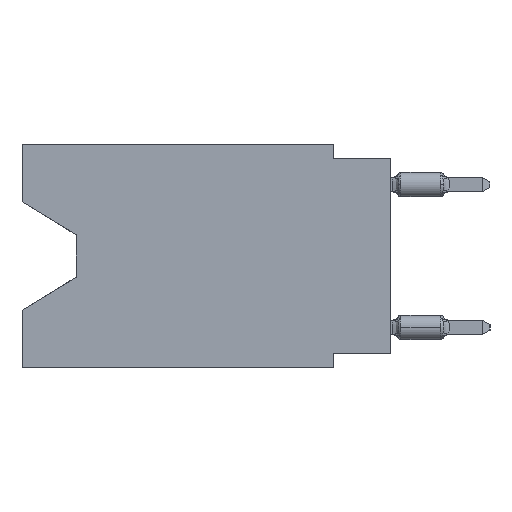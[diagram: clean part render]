
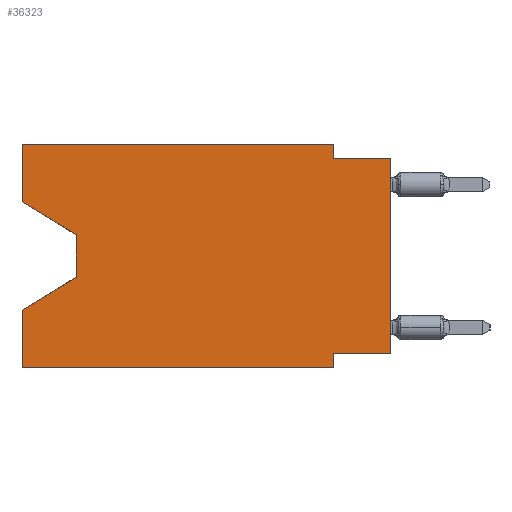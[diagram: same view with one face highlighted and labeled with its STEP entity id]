
A CAD part, left-side view. The second image highlights one B-rep face of the part: STEP entity #36323.
In plain terms, the highlighted planar face has unit normal (-1, 0, 0).
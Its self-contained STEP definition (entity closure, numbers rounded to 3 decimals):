
#800 = CARTESIAN_POINT ( 'NONE',  ( 0., 16.383, 0. ) ) ;
#2239 = LINE ( 'NONE', #11831, #48342 ) ;
#5700 = CARTESIAN_POINT ( 'NONE',  ( 0., 0., -0.635 ) ) ;
#6892 = CARTESIAN_POINT ( 'NONE',  ( 0., 16.383, 0. ) ) ;
#7285 = EDGE_CURVE ( 'NONE', #55213, #67198, #36756, .T. ) ;
#11448 = DIRECTION ( 'NONE',  ( 0., 0., -1. ) ) ;
#11802 = CARTESIAN_POINT ( 'NONE',  ( 0., 13.97, -5.893 ) ) ;
#11831 = CARTESIAN_POINT ( 'NONE',  ( 0., 0., 0. ) ) ;
#11960 = DIRECTION ( 'NONE',  ( 0., -1., 0. ) ) ;
#12684 = EDGE_CURVE ( 'NONE', #23240, #52207, #2239, .T. ) ;
#12736 = DIRECTION ( 'NONE',  ( 0., 1., 0. ) ) ;
#13069 = CARTESIAN_POINT ( 'NONE',  ( 0., 0., -9.271 ) ) ;
#14661 = VECTOR ( 'NONE', #11448, 1000. ) ;
#14761 = VECTOR ( 'NONE', #53350, 1000. ) ;
#14791 = VECTOR ( 'NONE', #12736, 1000. ) ;
#15826 = EDGE_CURVE ( 'NONE', #63662, #47888, #22528, .T. ) ;
#17516 = DIRECTION ( 'NONE',  ( 1., 0., 0. ) ) ;
#18167 = CARTESIAN_POINT ( 'NONE',  ( 0., 0., -0.635 ) ) ;
#18464 = VECTOR ( 'NONE', #56371, 1000. ) ;
#18908 = VECTOR ( 'NONE', #11960, 1000. ) ;
#19835 = VERTEX_POINT ( 'NONE', #65864 ) ;
#21396 = ORIENTED_EDGE ( 'NONE', *, *, #31389, .F. ) ;
#21735 = CARTESIAN_POINT ( 'NONE',  ( 0., 2.54, -9.906 ) ) ;
#22528 = LINE ( 'NONE', #32467, #14761 ) ;
#22677 = LINE ( 'NONE', #800, #52258 ) ;
#23240 = VERTEX_POINT ( 'NONE', #43966 ) ;
#23851 = CARTESIAN_POINT ( 'NONE',  ( 0., 13.97, -5.893 ) ) ;
#24217 = CARTESIAN_POINT ( 'NONE',  ( 0., 13.97, -4.013 ) ) ;
#25348 = EDGE_LOOP ( 'NONE', ( #44290, #29665, #33543, #37203, #29110, #52656, #36316, #64169, #21396, #58352, #28528, #28269 ) ) ;
#25919 = VERTEX_POINT ( 'NONE', #48844 ) ;
#27871 = LINE ( 'NONE', #37817, #14661 ) ;
#28008 = EDGE_CURVE ( 'NONE', #23240, #52487, #64433, .T. ) ;
#28269 = ORIENTED_EDGE ( 'NONE', *, *, #47150, .F. ) ;
#28528 = ORIENTED_EDGE ( 'NONE', *, *, #7285, .F. ) ;
#29110 = ORIENTED_EDGE ( 'NONE', *, *, #40261, .T. ) ;
#29665 = ORIENTED_EDGE ( 'NONE', *, *, #15826, .T. ) ;
#29707 = VECTOR ( 'NONE', #60527, 1000. ) ;
#31389 = EDGE_CURVE ( 'NONE', #46393, #52207, #39395, .T. ) ;
#31607 = CARTESIAN_POINT ( 'NONE',  ( 0., 16.383, 0. ) ) ;
#32467 = CARTESIAN_POINT ( 'NONE',  ( 0., 13.97, -4.013 ) ) ;
#32497 = VECTOR ( 'NONE', #43721, 1000. ) ;
#32940 = DIRECTION ( 'NONE',  ( 0., 0., 1. ) ) ;
#33543 = ORIENTED_EDGE ( 'NONE', *, *, #49444, .T. ) ;
#33613 = CARTESIAN_POINT ( 'NONE',  ( 0., 16.383, 0. ) ) ;
#33889 = EDGE_CURVE ( 'NONE', #19835, #63662, #44783, .T. ) ;
#34357 = CARTESIAN_POINT ( 'NONE',  ( 0., 16.383, -7.36 ) ) ;
#35207 = LINE ( 'NONE', #56763, #59615 ) ;
#35753 = VERTEX_POINT ( 'NONE', #21735 ) ;
#36316 = ORIENTED_EDGE ( 'NONE', *, *, #28008, .F. ) ;
#36323 = ADVANCED_FACE ( 'NONE', ( #38090 ), #58961, .F. ) ;
#36756 = LINE ( 'NONE', #31607, #66959 ) ;
#37203 = ORIENTED_EDGE ( 'NONE', *, *, #61105, .F. ) ;
#37817 = CARTESIAN_POINT ( 'NONE',  ( 0., 2.54, 0. ) ) ;
#37995 = CARTESIAN_POINT ( 'NONE',  ( 0., 16.383, -9.906 ) ) ;
#38090 = FACE_OUTER_BOUND ( 'NONE', #25348, .T. ) ;
#39395 = LINE ( 'NONE', #18167, #67564 ) ;
#40261 = EDGE_CURVE ( 'NONE', #25919, #35753, #58865, .T. ) ;
#41726 = EDGE_CURVE ( 'NONE', #67198, #46393, #27871, .T. ) ;
#43721 = DIRECTION ( 'NONE',  ( 0., 0.855, -0.519 ) ) ;
#43856 = DIRECTION ( 'NONE',  ( 0., -1., 0. ) ) ;
#43966 = CARTESIAN_POINT ( 'NONE',  ( 0., 0., -9.271 ) ) ;
#44290 = ORIENTED_EDGE ( 'NONE', *, *, #33889, .T. ) ;
#44783 = LINE ( 'NONE', #65651, #29707 ) ;
#46393 = VERTEX_POINT ( 'NONE', #66174 ) ;
#47150 = EDGE_CURVE ( 'NONE', #19835, #55213, #35207, .T. ) ;
#47888 = VERTEX_POINT ( 'NONE', #11802 ) ;
#48342 = VECTOR ( 'NONE', #64863, 1000. ) ;
#48371 = DIRECTION ( 'NONE',  ( 0., -1., 0. ) ) ;
#48844 = CARTESIAN_POINT ( 'NONE',  ( 0., 16.383, -9.906 ) ) ;
#49444 = EDGE_CURVE ( 'NONE', #47888, #59619, #59459, .T. ) ;
#52207 = VERTEX_POINT ( 'NONE', #5700 ) ;
#52258 = VECTOR ( 'NONE', #32940, 1000. ) ;
#52487 = VERTEX_POINT ( 'NONE', #61425 ) ;
#52656 = ORIENTED_EDGE ( 'NONE', *, *, #62608, .F. ) ;
#53350 = DIRECTION ( 'NONE',  ( 0., 0., -1. ) ) ;
#54489 = DIRECTION ( 'NONE',  ( 0., 0., -1. ) ) ;
#55213 = VERTEX_POINT ( 'NONE', #6892 ) ;
#56371 = DIRECTION ( 'NONE',  ( 0., 0., -1. ) ) ;
#56763 = CARTESIAN_POINT ( 'NONE',  ( 0., 16.383, 0. ) ) ;
#58352 = ORIENTED_EDGE ( 'NONE', *, *, #41726, .F. ) ;
#58865 = LINE ( 'NONE', #37995, #18908 ) ;
#58961 = PLANE ( 'NONE',  #64783 ) ;
#59459 = LINE ( 'NONE', #23851, #32497 ) ;
#59615 = VECTOR ( 'NONE', #61555, 1000. ) ;
#59619 = VERTEX_POINT ( 'NONE', #34357 ) ;
#60527 = DIRECTION ( 'NONE',  ( 0., -0.855, -0.519 ) ) ;
#61105 = EDGE_CURVE ( 'NONE', #25919, #59619, #22677, .T. ) ;
#61195 = CARTESIAN_POINT ( 'NONE',  ( 0., 2.54, 0. ) ) ;
#61425 = CARTESIAN_POINT ( 'NONE',  ( 0., 2.54, -9.271 ) ) ;
#61555 = DIRECTION ( 'NONE',  ( 0., 0., 1. ) ) ;
#61842 = CARTESIAN_POINT ( 'NONE',  ( 0., 2.54, -9.906 ) ) ;
#62608 = EDGE_CURVE ( 'NONE', #52487, #35753, #66293, .T. ) ;
#63662 = VERTEX_POINT ( 'NONE', #24217 ) ;
#64169 = ORIENTED_EDGE ( 'NONE', *, *, #12684, .T. ) ;
#64433 = LINE ( 'NONE', #13069, #14791 ) ;
#64783 = AXIS2_PLACEMENT_3D ( 'NONE', #33613, #17516, #54489 ) ;
#64863 = DIRECTION ( 'NONE',  ( 0., 0., 1. ) ) ;
#65651 = CARTESIAN_POINT ( 'NONE',  ( 0., 16.383, -2.546 ) ) ;
#65864 = CARTESIAN_POINT ( 'NONE',  ( 0., 16.383, -2.546 ) ) ;
#66174 = CARTESIAN_POINT ( 'NONE',  ( 0., 2.54, -0.635 ) ) ;
#66293 = LINE ( 'NONE', #61842, #18464 ) ;
#66959 = VECTOR ( 'NONE', #48371, 1000. ) ;
#67198 = VERTEX_POINT ( 'NONE', #61195 ) ;
#67564 = VECTOR ( 'NONE', #43856, 1000. ) ;
